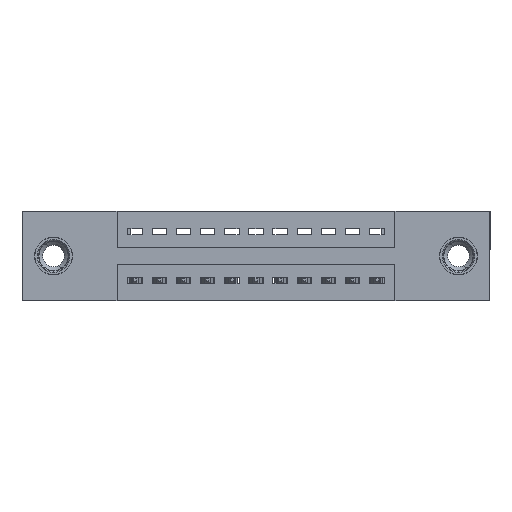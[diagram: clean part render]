
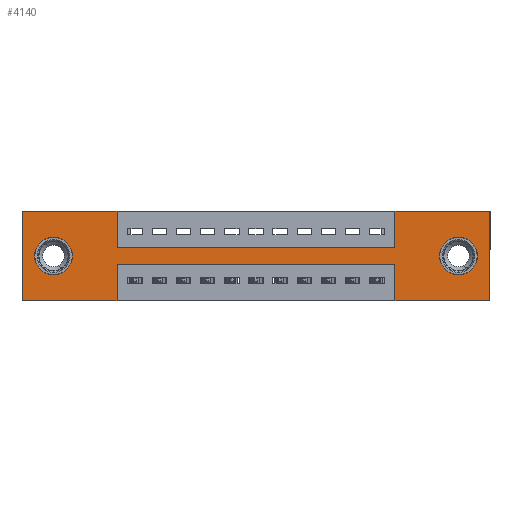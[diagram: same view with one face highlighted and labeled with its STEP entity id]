
A CAD part, front view. The second image highlights one B-rep face of the part: STEP entity #4140.
In plain terms, the highlighted planar face has unit normal (0, -1, 0).
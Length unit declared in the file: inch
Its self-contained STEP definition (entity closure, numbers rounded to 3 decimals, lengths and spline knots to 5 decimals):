
#167 = VECTOR ( 'NONE', #17227, 39.37008 ) ;
#184 = AXIS2_PLACEMENT_3D ( 'NONE', #9798, #9744, #12322 ) ;
#200 = ORIENTED_EDGE ( 'NONE', *, *, #15171, .T. ) ;
#485 = CARTESIAN_POINT ( 'NONE',  ( 1.805, 0., -0.107 ) ) ;
#513 = DIRECTION ( 'NONE',  ( 0., 0., -1. ) ) ;
#702 = DIRECTION ( 'NONE',  ( 0., 1., 0. ) ) ;
#738 = CARTESIAN_POINT ( 'NONE',  ( 1.5425, 0., -0.37 ) ) ;
#861 = CARTESIAN_POINT ( 'NONE',  ( 0., 0., -0.37 ) ) ;
#1070 = DIRECTION ( 'NONE',  ( 0., 0., 1. ) ) ;
#1092 = VECTOR ( 'NONE', #7811, 39.37008 ) ;
#1462 = CARTESIAN_POINT ( 'NONE',  ( 1.935, 0., 0. ) ) ;
#1604 = CARTESIAN_POINT ( 'NONE',  ( 1.5425, 0., 0. ) ) ;
#1724 = VERTEX_POINT ( 'NONE', #16023 ) ;
#1744 = FACE_BOUND ( 'NONE', #15419, .T. ) ;
#1798 = LINE ( 'NONE', #5785, #12032 ) ;
#1883 = DIRECTION ( 'NONE',  ( -1., 0., 0. ) ) ;
#1915 = EDGE_CURVE ( 'NONE', #16766, #11043, #9312, .T. ) ;
#2023 = CIRCLE ( 'NONE', #7033, 0.078 ) ;
#2054 = DIRECTION ( 'NONE',  ( 0., 0., -1. ) ) ;
#2147 = CARTESIAN_POINT ( 'NONE',  ( 0., 0., -0.37 ) ) ;
#2191 = CARTESIAN_POINT ( 'NONE',  ( 0., 0., 0. ) ) ;
#2334 = LINE ( 'NONE', #1604, #10666 ) ;
#2412 = ORIENTED_EDGE ( 'NONE', *, *, #8906, .F. ) ;
#2616 = VECTOR ( 'NONE', #1883, 39.37008 ) ;
#2633 = EDGE_CURVE ( 'NONE', #11395, #10933, #11145, .T. ) ;
#2713 = CARTESIAN_POINT ( 'NONE',  ( 0., 0., 0. ) ) ;
#2751 = ORIENTED_EDGE ( 'NONE', *, *, #5637, .F. ) ;
#3317 = AXIS2_PLACEMENT_3D ( 'NONE', #7771, #13126, #14408 ) ;
#3381 = DIRECTION ( 'NONE',  ( -1., 0., 0. ) ) ;
#3403 = EDGE_CURVE ( 'NONE', #14194, #8662, #7818, .T. ) ;
#3858 = CARTESIAN_POINT ( 'NONE',  ( 0.3925, 0., -0.15 ) ) ;
#3892 = CARTESIAN_POINT ( 'NONE',  ( 0.13, 0., -0.185 ) ) ;
#3934 = CARTESIAN_POINT ( 'NONE',  ( 0., 0., 0. ) ) ;
#4136 = LINE ( 'NONE', #6015, #11645 ) ;
#4140 = ADVANCED_FACE ( 'NONE', ( #1744, #15244, #8220 ), #5319, .T. ) ;
#4208 = ORIENTED_EDGE ( 'NONE', *, *, #8656, .F. ) ;
#4378 = VERTEX_POINT ( 'NONE', #5691 ) ;
#4566 = VERTEX_POINT ( 'NONE', #16885 ) ;
#4696 = EDGE_CURVE ( 'NONE', #17076, #4378, #6755, .T. ) ;
#4805 = CARTESIAN_POINT ( 'NONE',  ( 1.5425, 0., 0. ) ) ;
#5038 = VECTOR ( 'NONE', #3381, 39.37008 ) ;
#5319 = PLANE ( 'NONE',  #3317 ) ;
#5595 = LINE ( 'NONE', #3934, #167 ) ;
#5637 = EDGE_CURVE ( 'NONE', #1724, #14194, #12379, .T. ) ;
#5649 = CARTESIAN_POINT ( 'NONE',  ( 0.3925, 0., -0.37 ) ) ;
#5691 = CARTESIAN_POINT ( 'NONE',  ( 1.5425, 0., -0.15 ) ) ;
#5755 = DIRECTION ( 'NONE',  ( 1., 0., 0. ) ) ;
#5785 = CARTESIAN_POINT ( 'NONE',  ( 1.5425, 0., -0.37 ) ) ;
#5909 = CARTESIAN_POINT ( 'NONE',  ( 0.3925, 0., 0. ) ) ;
#5917 = DIRECTION ( 'NONE',  ( 0., 0., 1. ) ) ;
#5946 = ORIENTED_EDGE ( 'NONE', *, *, #14928, .F. ) ;
#5965 = ORIENTED_EDGE ( 'NONE', *, *, #4696, .F. ) ;
#6015 = CARTESIAN_POINT ( 'NONE',  ( 1.935, 0., 0. ) ) ;
#6216 = AXIS2_PLACEMENT_3D ( 'NONE', #11389, #702, #6270 ) ;
#6270 = DIRECTION ( 'NONE',  ( 0., 0., -1. ) ) ;
#6303 = CARTESIAN_POINT ( 'NONE',  ( 0.3925, 0., -0.22 ) ) ;
#6429 = VECTOR ( 'NONE', #12813, 39.37008 ) ;
#6755 = LINE ( 'NONE', #9366, #1092 ) ;
#6796 = AXIS2_PLACEMENT_3D ( 'NONE', #9803, #16420, #5917 ) ;
#7033 = AXIS2_PLACEMENT_3D ( 'NONE', #3892, #13228, #15858 ) ;
#7139 = VERTEX_POINT ( 'NONE', #15383 ) ;
#7258 = ORIENTED_EDGE ( 'NONE', *, *, #1915, .F. ) ;
#7516 = VERTEX_POINT ( 'NONE', #738 ) ;
#7657 = EDGE_CURVE ( 'NONE', #4378, #9723, #2334, .T. ) ;
#7735 = EDGE_CURVE ( 'NONE', #15644, #7516, #16043, .T. ) ;
#7771 = CARTESIAN_POINT ( 'NONE',  ( 0., 0., -0.37 ) ) ;
#7811 = DIRECTION ( 'NONE',  ( 1., 0., 0. ) ) ;
#7818 = LINE ( 'NONE', #5649, #10915 ) ;
#8220 = FACE_OUTER_BOUND ( 'NONE', #12759, .T. ) ;
#8288 = CIRCLE ( 'NONE', #184, 0.078 ) ;
#8334 = ORIENTED_EDGE ( 'NONE', *, *, #3403, .F. ) ;
#8656 = EDGE_CURVE ( 'NONE', #14992, #16766, #12498, .T. ) ;
#8662 = VERTEX_POINT ( 'NONE', #17049 ) ;
#8675 = ORIENTED_EDGE ( 'NONE', *, *, #15752, .F. ) ;
#8848 = LINE ( 'NONE', #5909, #9477 ) ;
#8906 = EDGE_CURVE ( 'NONE', #13881, #15644, #4136, .T. ) ;
#9312 = LINE ( 'NONE', #13670, #15514 ) ;
#9366 = CARTESIAN_POINT ( 'NONE',  ( 0.3925, 0., -0.15 ) ) ;
#9477 = VECTOR ( 'NONE', #13931, 39.37008 ) ;
#9723 = VERTEX_POINT ( 'NONE', #4805 ) ;
#9733 = DIRECTION ( 'NONE',  ( 0., 0., 1. ) ) ;
#9744 = DIRECTION ( 'NONE',  ( 0., 1., 0. ) ) ;
#9754 = CARTESIAN_POINT ( 'NONE',  ( 1.935, 0., -0.37 ) ) ;
#9798 = CARTESIAN_POINT ( 'NONE',  ( 1.805, 0., -0.185 ) ) ;
#9803 = CARTESIAN_POINT ( 'NONE',  ( 0.13, 0., -0.185 ) ) ;
#10666 = VECTOR ( 'NONE', #1070, 39.37008 ) ;
#10747 = CARTESIAN_POINT ( 'NONE',  ( 0., 0., -0.37 ) ) ;
#10915 = VECTOR ( 'NONE', #2054, 39.37008 ) ;
#10933 = VERTEX_POINT ( 'NONE', #485 ) ;
#11043 = VERTEX_POINT ( 'NONE', #16219 ) ;
#11145 = CIRCLE ( 'NONE', #6216, 0.078 ) ;
#11201 = CARTESIAN_POINT ( 'NONE',  ( 0.3925, 0., -0.22 ) ) ;
#11389 = CARTESIAN_POINT ( 'NONE',  ( 1.805, 0., -0.185 ) ) ;
#11395 = VERTEX_POINT ( 'NONE', #12043 ) ;
#11427 = EDGE_CURVE ( 'NONE', #11043, #17076, #8848, .T. ) ;
#11645 = VECTOR ( 'NONE', #513, 39.37008 ) ;
#12032 = VECTOR ( 'NONE', #9733, 39.37008 ) ;
#12043 = CARTESIAN_POINT ( 'NONE',  ( 1.805, 0., -0.263 ) ) ;
#12322 = DIRECTION ( 'NONE',  ( 0., 0., -1. ) ) ;
#12379 = LINE ( 'NONE', #11201, #2616 ) ;
#12457 = ORIENTED_EDGE ( 'NONE', *, *, #7657, .F. ) ;
#12498 = LINE ( 'NONE', #2191, #15585 ) ;
#12759 = EDGE_LOOP ( 'NONE', ( #8334, #2751, #14380, #14716, #2412, #5946, #12457, #5965, #14958, #7258, #4208, #8675 ) ) ;
#12795 = EDGE_CURVE ( 'NONE', #4566, #7139, #15640, .T. ) ;
#12813 = DIRECTION ( 'NONE',  ( -1., 0., 0. ) ) ;
#13126 = DIRECTION ( 'NONE',  ( 0., -1., 0. ) ) ;
#13228 = DIRECTION ( 'NONE',  ( 0., 1., 0. ) ) ;
#13493 = LINE ( 'NONE', #2147, #6429 ) ;
#13670 = CARTESIAN_POINT ( 'NONE',  ( 0., 0., 0. ) ) ;
#13773 = EDGE_LOOP ( 'NONE', ( #16992, #16867 ) ) ;
#13881 = VERTEX_POINT ( 'NONE', #1462 ) ;
#13931 = DIRECTION ( 'NONE',  ( 0., 0., -1. ) ) ;
#14146 = DIRECTION ( 'NONE',  ( 0., 0., 1. ) ) ;
#14194 = VERTEX_POINT ( 'NONE', #6303 ) ;
#14380 = ORIENTED_EDGE ( 'NONE', *, *, #16208, .F. ) ;
#14408 = DIRECTION ( 'NONE',  ( 0., 0., -1. ) ) ;
#14716 = ORIENTED_EDGE ( 'NONE', *, *, #7735, .F. ) ;
#14928 = EDGE_CURVE ( 'NONE', #9723, #13881, #5595, .T. ) ;
#14958 = ORIENTED_EDGE ( 'NONE', *, *, #11427, .F. ) ;
#14992 = VERTEX_POINT ( 'NONE', #10747 ) ;
#15171 = EDGE_CURVE ( 'NONE', #10933, #11395, #8288, .T. ) ;
#15244 = FACE_BOUND ( 'NONE', #13773, .T. ) ;
#15383 = CARTESIAN_POINT ( 'NONE',  ( 0.13, 0., -0.107 ) ) ;
#15419 = EDGE_LOOP ( 'NONE', ( #200, #16545 ) ) ;
#15514 = VECTOR ( 'NONE', #5755, 39.37008 ) ;
#15585 = VECTOR ( 'NONE', #14146, 39.37008 ) ;
#15640 = CIRCLE ( 'NONE', #6796, 0.078 ) ;
#15644 = VERTEX_POINT ( 'NONE', #9754 ) ;
#15752 = EDGE_CURVE ( 'NONE', #8662, #14992, #13493, .T. ) ;
#15858 = DIRECTION ( 'NONE',  ( 0., 0., 1. ) ) ;
#15952 = EDGE_CURVE ( 'NONE', #7139, #4566, #2023, .T. ) ;
#16023 = CARTESIAN_POINT ( 'NONE',  ( 1.5425, 0., -0.22 ) ) ;
#16043 = LINE ( 'NONE', #861, #5038 ) ;
#16208 = EDGE_CURVE ( 'NONE', #7516, #1724, #1798, .T. ) ;
#16219 = CARTESIAN_POINT ( 'NONE',  ( 0.3925, 0., 0. ) ) ;
#16420 = DIRECTION ( 'NONE',  ( 0., 1., 0. ) ) ;
#16545 = ORIENTED_EDGE ( 'NONE', *, *, #2633, .T. ) ;
#16766 = VERTEX_POINT ( 'NONE', #2713 ) ;
#16867 = ORIENTED_EDGE ( 'NONE', *, *, #12795, .T. ) ;
#16885 = CARTESIAN_POINT ( 'NONE',  ( 0.13, 0., -0.263 ) ) ;
#16992 = ORIENTED_EDGE ( 'NONE', *, *, #15952, .T. ) ;
#17049 = CARTESIAN_POINT ( 'NONE',  ( 0.3925, 0., -0.37 ) ) ;
#17076 = VERTEX_POINT ( 'NONE', #3858 ) ;
#17227 = DIRECTION ( 'NONE',  ( 1., 0., 0. ) ) ;
